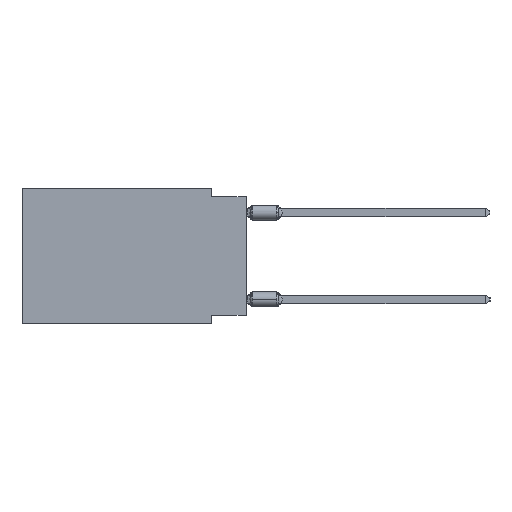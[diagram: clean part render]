
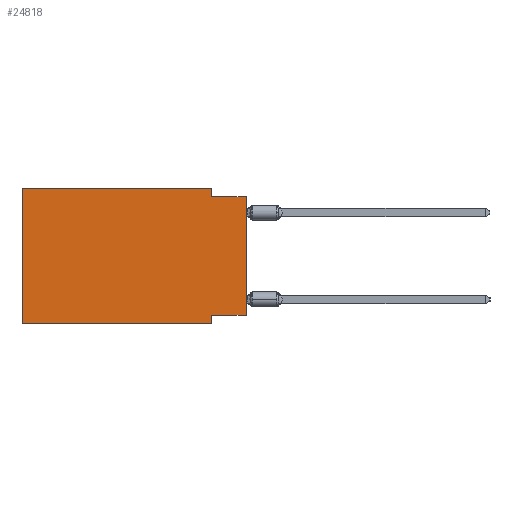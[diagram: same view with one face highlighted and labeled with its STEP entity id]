
A CAD part, left-side view. The second image highlights one B-rep face of the part: STEP entity #24818.
In plain terms, the highlighted planar face has unit normal (-1, 0, 0).
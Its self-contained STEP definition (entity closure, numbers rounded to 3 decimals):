
#316 = AXIS2_PLACEMENT_3D ( 'NONE', #21407, #41384, #38053 ) ;
#965 = CARTESIAN_POINT ( 'NONE',  ( 0., 16.383, -9.906 ) ) ;
#1008 = VECTOR ( 'NONE', #34530, 1000. ) ;
#1579 = VECTOR ( 'NONE', #7824, 1000. ) ;
#2209 = ORIENTED_EDGE ( 'NONE', *, *, #17478, .F. ) ;
#2760 = LINE ( 'NONE', #30241, #19422 ) ;
#3145 = CARTESIAN_POINT ( 'NONE',  ( 0., 2.54, -9.271 ) ) ;
#4118 = CARTESIAN_POINT ( 'NONE',  ( 0., 2.54, 0. ) ) ;
#4239 = VECTOR ( 'NONE', #26876, 1000. ) ;
#4386 = VERTEX_POINT ( 'NONE', #28271 ) ;
#4660 = VECTOR ( 'NONE', #28348, 1000. ) ;
#4943 = ORIENTED_EDGE ( 'NONE', *, *, #35517, .F. ) ;
#5331 = EDGE_CURVE ( 'NONE', #4386, #21967, #40045, .T. ) ;
#7279 = LINE ( 'NONE', #17906, #1008 ) ;
#7824 = DIRECTION ( 'NONE',  ( 0., 0., 1. ) ) ;
#10828 = CARTESIAN_POINT ( 'NONE',  ( 0., 2.54, 0. ) ) ;
#11460 = CARTESIAN_POINT ( 'NONE',  ( 0., 16.383, -9.906 ) ) ;
#11590 = CARTESIAN_POINT ( 'NONE',  ( 0., 0., 0. ) ) ;
#11604 = VECTOR ( 'NONE', #29854, 1000. ) ;
#13706 = ORIENTED_EDGE ( 'NONE', *, *, #24396, .F. ) ;
#14121 = EDGE_CURVE ( 'NONE', #20291, #21967, #41517, .T. ) ;
#16720 = EDGE_CURVE ( 'NONE', #17007, #19468, #21100, .T. ) ;
#17007 = VERTEX_POINT ( 'NONE', #11460 ) ;
#17478 = EDGE_CURVE ( 'NONE', #35617, #4386, #38017, .T. ) ;
#17850 = CARTESIAN_POINT ( 'NONE',  ( 0., 16.383, 0. ) ) ;
#17906 = CARTESIAN_POINT ( 'NONE',  ( 0., 0., -9.271 ) ) ;
#18297 = CARTESIAN_POINT ( 'NONE',  ( 0., 2.54, -9.906 ) ) ;
#18309 = PLANE ( 'NONE',  #316 ) ;
#19422 = VECTOR ( 'NONE', #20028, 1000. ) ;
#19468 = VERTEX_POINT ( 'NONE', #18297 ) ;
#20028 = DIRECTION ( 'NONE',  ( 0., 0., 1. ) ) ;
#20291 = VERTEX_POINT ( 'NONE', #28400 ) ;
#21100 = LINE ( 'NONE', #965, #4239 ) ;
#21407 = CARTESIAN_POINT ( 'NONE',  ( 0., 16.383, 0. ) ) ;
#21942 = LINE ( 'NONE', #35463, #11604 ) ;
#21967 = VERTEX_POINT ( 'NONE', #29454 ) ;
#22741 = ORIENTED_EDGE ( 'NONE', *, *, #37494, .F. ) ;
#24396 = EDGE_CURVE ( 'NONE', #34984, #19468, #25247, .T. ) ;
#24818 = ADVANCED_FACE ( 'NONE', ( #34940 ), #18309, .F. ) ;
#24920 = ORIENTED_EDGE ( 'NONE', *, *, #5331, .F. ) ;
#25247 = LINE ( 'NONE', #35418, #4660 ) ;
#26876 = DIRECTION ( 'NONE',  ( 0., -1., 0. ) ) ;
#28271 = CARTESIAN_POINT ( 'NONE',  ( 0., 2.54, -0.635 ) ) ;
#28348 = DIRECTION ( 'NONE',  ( 0., 0., -1. ) ) ;
#28400 = CARTESIAN_POINT ( 'NONE',  ( 0., 0., -9.271 ) ) ;
#29454 = CARTESIAN_POINT ( 'NONE',  ( 0., 0., -0.635 ) ) ;
#29854 = DIRECTION ( 'NONE',  ( 0., -1., 0. ) ) ;
#30080 = DIRECTION ( 'NONE',  ( 0., -1., 0. ) ) ;
#30241 = CARTESIAN_POINT ( 'NONE',  ( 0., 16.383, 0. ) ) ;
#32638 = VECTOR ( 'NONE', #34250, 1000. ) ;
#32778 = VERTEX_POINT ( 'NONE', #17850 ) ;
#34250 = DIRECTION ( 'NONE',  ( 0., 0., -1. ) ) ;
#34530 = DIRECTION ( 'NONE',  ( 0., 1., 0. ) ) ;
#34940 = FACE_OUTER_BOUND ( 'NONE', #37439, .T. ) ;
#34984 = VERTEX_POINT ( 'NONE', #3145 ) ;
#35418 = CARTESIAN_POINT ( 'NONE',  ( 0., 2.54, -9.906 ) ) ;
#35463 = CARTESIAN_POINT ( 'NONE',  ( 0., 16.383, 0. ) ) ;
#35517 = EDGE_CURVE ( 'NONE', #20291, #34984, #7279, .T. ) ;
#35617 = VERTEX_POINT ( 'NONE', #10828 ) ;
#36140 = VECTOR ( 'NONE', #30080, 1000. ) ;
#36709 = CARTESIAN_POINT ( 'NONE',  ( 0., 0., -0.635 ) ) ;
#37439 = EDGE_LOOP ( 'NONE', ( #38896, #24920, #2209, #40226, #22741, #38343, #13706, #4943 ) ) ;
#37494 = EDGE_CURVE ( 'NONE', #17007, #32778, #2760, .T. ) ;
#38017 = LINE ( 'NONE', #4118, #32638 ) ;
#38053 = DIRECTION ( 'NONE',  ( 0., 0., -1. ) ) ;
#38343 = ORIENTED_EDGE ( 'NONE', *, *, #16720, .T. ) ;
#38896 = ORIENTED_EDGE ( 'NONE', *, *, #14121, .T. ) ;
#40045 = LINE ( 'NONE', #36709, #36140 ) ;
#40226 = ORIENTED_EDGE ( 'NONE', *, *, #41785, .F. ) ;
#41384 = DIRECTION ( 'NONE',  ( 1., 0., 0. ) ) ;
#41517 = LINE ( 'NONE', #11590, #1579 ) ;
#41785 = EDGE_CURVE ( 'NONE', #32778, #35617, #21942, .T. ) ;
